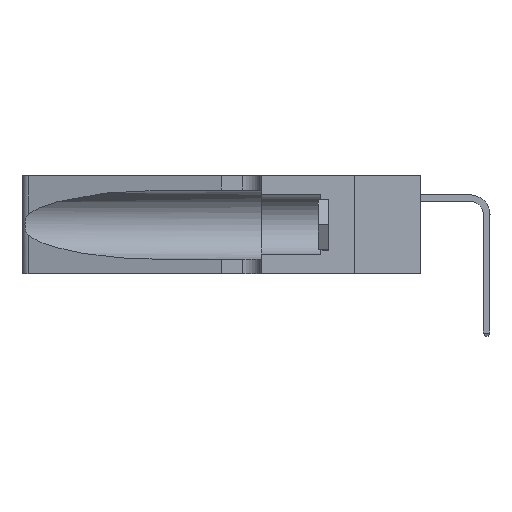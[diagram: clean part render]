
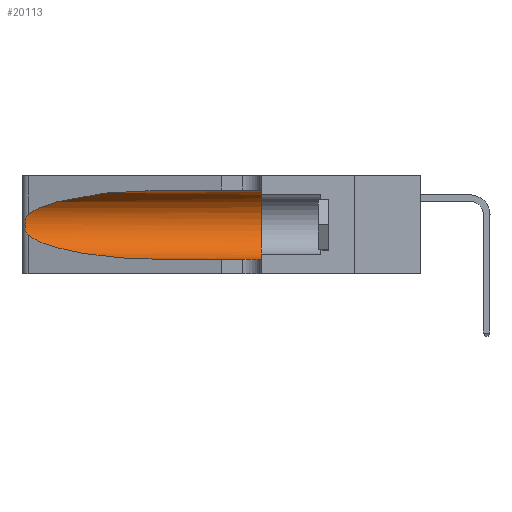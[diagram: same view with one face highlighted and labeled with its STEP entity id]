
A CAD part, left-side view. The second image highlights one B-rep face of the part: STEP entity #20113.
In plain terms, the highlighted cylindrical face has radius 3.308 mm (diameter 6.617 mm), a partial arc.
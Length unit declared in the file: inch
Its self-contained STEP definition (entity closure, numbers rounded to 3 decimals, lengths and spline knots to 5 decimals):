
#129 = VECTOR ( 'NONE', #23201, 39.37008 ) ;
#1204 = LINE ( 'NONE', #26404, #129 ) ;
#1539 = CARTESIAN_POINT ( 'NONE',  ( 0.26075, 1.23896, 0.178 ) ) ;
#2558 = CARTESIAN_POINT ( 'NONE',  ( 0.1305, 0.72297, 0.05475 ) ) ;
#3075 = VERTEX_POINT ( 'NONE', #20978 ) ;
#4517 = CYLINDRICAL_SURFACE ( 'NONE', #31244, 0.13025 ) ;
#4805 = EDGE_LOOP ( 'NONE', ( #25509, #25911, #33470, #7905, #39912, #28604 ) ) ;
#4849 = CARTESIAN_POINT ( 'NONE',  ( 0.25487, 1.22718, 0.22369 ) ) ;
#4967 = VERTEX_POINT ( 'NONE', #7495 ) ;
#5001 = CARTESIAN_POINT ( 'NONE',  ( 0.25856, 1.23593, 0.16098 ) ) ;
#5787 = CIRCLE ( 'NONE', #26926, 0.13025 ) ;
#6288 = B_SPLINE_CURVE_WITH_KNOTS ( 'NONE', 3,
 ( #4849, #25147, #15066, #38613, #18475, #41996, #21931, #1539, #25290, #5001, #28678, #8432, #32063, #11802 ),
 .UNSPECIFIED., .F., .F.,
 ( 4, 2, 2, 2, 2, 2, 4 ),
 ( 0., 0.00027, 0.00053, 0.00107, 0.0016, 0.00187, 0.00214 ),
 .UNSPECIFIED. ) ;
#6415 = CARTESIAN_POINT ( 'NONE',  ( 0.2373, 1.15595, 0.28018 ) ) ;
#7495 = CARTESIAN_POINT ( 'NONE',  ( 0.1305, 0.35, 0.05475 ) ) ;
#7905 = ORIENTED_EDGE ( 'NONE', *, *, #21772, .T. ) ;
#8432 = CARTESIAN_POINT ( 'NONE',  ( 0.25639, 1.23186, 0.15144 ) ) ;
#9282 = CARTESIAN_POINT ( 'NONE',  ( 0.25487, 1.22718, 0.14631 ) ) ;
#10766 = DIRECTION ( 'NONE',  ( 0., 0., -1. ) ) ;
#10822 =( BOUNDED_CURVE ( )  B_SPLINE_CURVE ( 3, ( #23289, #19874, #6415, #30041 ),
 .UNSPECIFIED., .F., .T. ) 
 B_SPLINE_CURVE_WITH_KNOTS ( ( 4, 4 ),
 ( 1.5708, 2.84003 ),
 .UNSPECIFIED. ) 
 CURVE ( )  GEOMETRIC_REPRESENTATION_ITEM ( )  RATIONAL_B_SPLINE_CURVE ( ( 1., 0.87, 0.87, 1. ) ) 
 REPRESENTATION_ITEM ( '' )  );
#11448 = CARTESIAN_POINT ( 'NONE',  ( 0.1305, 0.35, 0.185 ) ) ;
#11802 = CARTESIAN_POINT ( 'NONE',  ( 0.25487, 1.22718, 0.14631 ) ) ;
#12856 = VERTEX_POINT ( 'NONE', #32696 ) ;
#14844 = DIRECTION ( 'NONE',  ( 0., 0., 1. ) ) ;
#14919 = VERTEX_POINT ( 'NONE', #37528 ) ;
#15066 = CARTESIAN_POINT ( 'NONE',  ( 0.25639, 1.23184, 0.21858 ) ) ;
#15402 = EDGE_CURVE ( 'NONE', #40492, #3075, #10822, .T. ) ;
#17532 = CARTESIAN_POINT ( 'NONE',  ( 0.1305, 0.35, 0.31525 ) ) ;
#18475 = CARTESIAN_POINT ( 'NONE',  ( 0.25854, 1.2359, 0.20912 ) ) ;
#18616 =( BOUNDED_CURVE ( )  B_SPLINE_CURVE ( 3, ( #9282, #29536, #22937, #2558 ),
 .UNSPECIFIED., .F., .F. ) 
 B_SPLINE_CURVE_WITH_KNOTS ( ( 4, 4 ),
 ( 3.44316, 4.71239 ),
 .UNSPECIFIED. ) 
 CURVE ( )  GEOMETRIC_REPRESENTATION_ITEM ( )  RATIONAL_B_SPLINE_CURVE ( ( 1., 0.87, 0.87, 1. ) ) 
 REPRESENTATION_ITEM ( '' )  );
#19874 = CARTESIAN_POINT ( 'NONE',  ( 0.18966, 0.96281, 0.31525 ) ) ;
#20113 = ADVANCED_FACE ( 'NONE', ( #22595 ), #4517, .F. ) ;
#20888 = DIRECTION ( 'NONE',  ( 0., -1., 0. ) ) ;
#20978 = CARTESIAN_POINT ( 'NONE',  ( 0.25487, 1.22718, 0.22369 ) ) ;
#21772 = EDGE_CURVE ( 'NONE', #12856, #4967, #1204, .T. ) ;
#21931 = CARTESIAN_POINT ( 'NONE',  ( 0.26075, 1.23896, 0.19203 ) ) ;
#22410 = EDGE_CURVE ( 'NONE', #40492, #32848, #35522, .T. ) ;
#22595 = FACE_OUTER_BOUND ( 'NONE', #4805, .T. ) ;
#22788 = EDGE_CURVE ( 'NONE', #3075, #14919, #6288, .T. ) ;
#22937 = CARTESIAN_POINT ( 'NONE',  ( 0.18966, 0.96281, 0.05475 ) ) ;
#23201 = DIRECTION ( 'NONE',  ( 0., -1., 0. ) ) ;
#23289 = CARTESIAN_POINT ( 'NONE',  ( 0.1305, 0.72297, 0.31525 ) ) ;
#25147 = CARTESIAN_POINT ( 'NONE',  ( 0.25555, 1.22994, 0.2215 ) ) ;
#25290 = CARTESIAN_POINT ( 'NONE',  ( 0.26017, 1.23833, 0.17102 ) ) ;
#25509 = ORIENTED_EDGE ( 'NONE', *, *, #15402, .T. ) ;
#25569 = VECTOR ( 'NONE', #30036, 39.37008 ) ;
#25911 = ORIENTED_EDGE ( 'NONE', *, *, #22788, .T. ) ;
#26404 = CARTESIAN_POINT ( 'NONE',  ( 0.1305, 1.61858, 0.05475 ) ) ;
#26926 = AXIS2_PLACEMENT_3D ( 'NONE', #11448, #35027, #14844 ) ;
#28604 = ORIENTED_EDGE ( 'NONE', *, *, #22410, .F. ) ;
#28678 = CARTESIAN_POINT ( 'NONE',  ( 0.25789, 1.23486, 0.15765 ) ) ;
#29111 = CARTESIAN_POINT ( 'NONE',  ( 0.1305, 0.72297, 0.31525 ) ) ;
#29536 = CARTESIAN_POINT ( 'NONE',  ( 0.2373, 1.15595, 0.08982 ) ) ;
#30036 = DIRECTION ( 'NONE',  ( 0., -1., 0. ) ) ;
#30041 = CARTESIAN_POINT ( 'NONE',  ( 0.25487, 1.22718, 0.22369 ) ) ;
#31016 = CARTESIAN_POINT ( 'NONE',  ( 0.1305, 1.61858, 0.185 ) ) ;
#31244 = AXIS2_PLACEMENT_3D ( 'NONE', #31016, #20888, #10766 ) ;
#31722 = EDGE_CURVE ( 'NONE', #14919, #12856, #18616, .T. ) ;
#32063 = CARTESIAN_POINT ( 'NONE',  ( 0.25555, 1.22993, 0.14849 ) ) ;
#32696 = CARTESIAN_POINT ( 'NONE',  ( 0.1305, 0.72297, 0.05475 ) ) ;
#32848 = VERTEX_POINT ( 'NONE', #17532 ) ;
#33470 = ORIENTED_EDGE ( 'NONE', *, *, #31722, .T. ) ;
#35027 = DIRECTION ( 'NONE',  ( 0., 1., 0. ) ) ;
#35522 = LINE ( 'NONE', #43322, #25569 ) ;
#37528 = CARTESIAN_POINT ( 'NONE',  ( 0.25487, 1.22718, 0.14631 ) ) ;
#38613 = CARTESIAN_POINT ( 'NONE',  ( 0.25787, 1.23484, 0.2124 ) ) ;
#39147 = EDGE_CURVE ( 'NONE', #32848, #4967, #5787, .T. ) ;
#39912 = ORIENTED_EDGE ( 'NONE', *, *, #39147, .F. ) ;
#40492 = VERTEX_POINT ( 'NONE', #29111 ) ;
#41996 = CARTESIAN_POINT ( 'NONE',  ( 0.26018, 1.23835, 0.19895 ) ) ;
#43322 = CARTESIAN_POINT ( 'NONE',  ( 0.1305, 1.61858, 0.31525 ) ) ;
